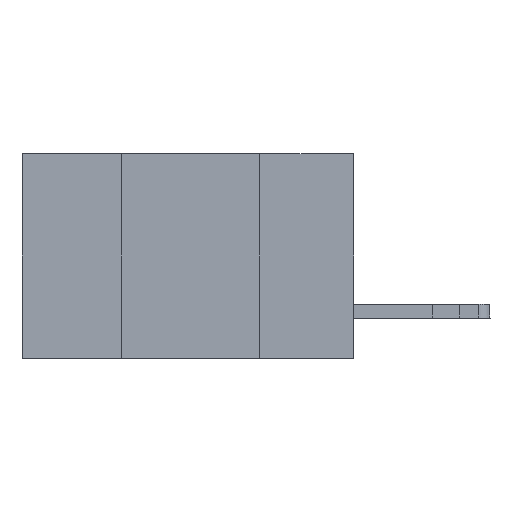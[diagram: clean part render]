
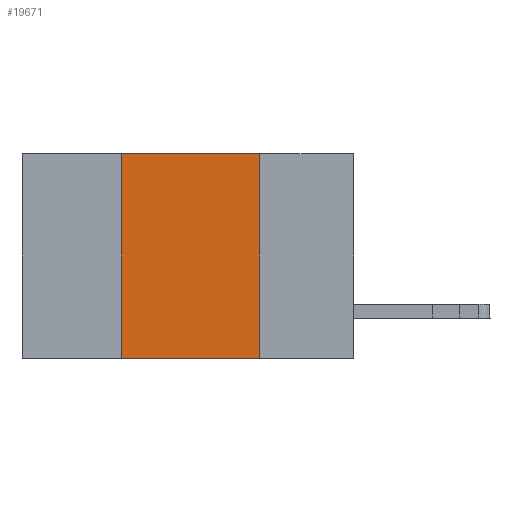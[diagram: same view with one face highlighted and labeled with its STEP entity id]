
A CAD part, left-side view. The second image highlights one B-rep face of the part: STEP entity #19671.
In plain terms, the highlighted planar face has unit normal (-1, 0, 0).
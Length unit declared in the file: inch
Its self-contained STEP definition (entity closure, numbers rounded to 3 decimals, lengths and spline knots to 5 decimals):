
#10 = VERTEX_POINT ( 'NONE', #20127 ) ;
#370 = CARTESIAN_POINT ( 'NONE',  ( 0., 0.17, 0. ) ) ;
#1012 = VECTOR ( 'NONE', #22702, 39.37008 ) ;
#1130 = EDGE_CURVE ( 'NONE', #22277, #26753, #24976, .T. ) ;
#1258 = CARTESIAN_POINT ( 'NONE',  ( 0., 0.17, 0. ) ) ;
#2277 = EDGE_LOOP ( 'NONE', ( #14305, #7142, #12013, #11445 ) ) ;
#2463 = DIRECTION ( 'NONE',  ( 0., 0., -1. ) ) ;
#4922 = VERTEX_POINT ( 'NONE', #370 ) ;
#5889 = LINE ( 'NONE', #12226, #25338 ) ;
#7142 = ORIENTED_EDGE ( 'NONE', *, *, #27469, .F. ) ;
#8531 = CARTESIAN_POINT ( 'NONE',  ( 0., 0.17, -0.37 ) ) ;
#10058 = VECTOR ( 'NONE', #18315, 39.37008 ) ;
#10457 = DIRECTION ( 'NONE',  ( 0., -1., 0. ) ) ;
#11445 = ORIENTED_EDGE ( 'NONE', *, *, #1130, .T. ) ;
#12001 = LINE ( 'NONE', #14107, #1012 ) ;
#12013 = ORIENTED_EDGE ( 'NONE', *, *, #21006, .F. ) ;
#12226 = CARTESIAN_POINT ( 'NONE',  ( 0., 0.42, 0. ) ) ;
#14107 = CARTESIAN_POINT ( 'NONE',  ( 0., 0.6, 0. ) ) ;
#14212 = EDGE_CURVE ( 'NONE', #4922, #26753, #20287, .T. ) ;
#14305 = ORIENTED_EDGE ( 'NONE', *, *, #14212, .F. ) ;
#14518 = CARTESIAN_POINT ( 'NONE',  ( 0., 0.6, -0.37 ) ) ;
#15742 = CARTESIAN_POINT ( 'NONE',  ( 0., 0.6, 0. ) ) ;
#16024 = PLANE ( 'NONE',  #24983 ) ;
#18104 = FACE_OUTER_BOUND ( 'NONE', #2277, .T. ) ;
#18136 = VECTOR ( 'NONE', #10457, 39.37008 ) ;
#18315 = DIRECTION ( 'NONE',  ( 0., 0., -1. ) ) ;
#19671 = ADVANCED_FACE ( 'NONE', ( #18104 ), #16024, .F. ) ;
#20127 = CARTESIAN_POINT ( 'NONE',  ( 0., 0.42, 0. ) ) ;
#20287 = LINE ( 'NONE', #1258, #10058 ) ;
#20940 = DIRECTION ( 'NONE',  ( 0., 0., 1. ) ) ;
#21006 = EDGE_CURVE ( 'NONE', #22277, #10, #5889, .T. ) ;
#22277 = VERTEX_POINT ( 'NONE', #25342 ) ;
#22702 = DIRECTION ( 'NONE',  ( 0., -1., 0. ) ) ;
#24491 = DIRECTION ( 'NONE',  ( 1., 0., 0. ) ) ;
#24976 = LINE ( 'NONE', #14518, #18136 ) ;
#24983 = AXIS2_PLACEMENT_3D ( 'NONE', #15742, #24491, #2463 ) ;
#25338 = VECTOR ( 'NONE', #20940, 39.37008 ) ;
#25342 = CARTESIAN_POINT ( 'NONE',  ( 0., 0.42, -0.37 ) ) ;
#26753 = VERTEX_POINT ( 'NONE', #8531 ) ;
#27469 = EDGE_CURVE ( 'NONE', #10, #4922, #12001, .T. ) ;
